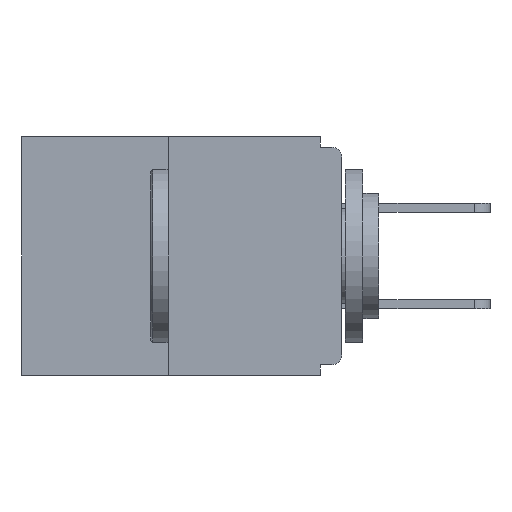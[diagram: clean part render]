
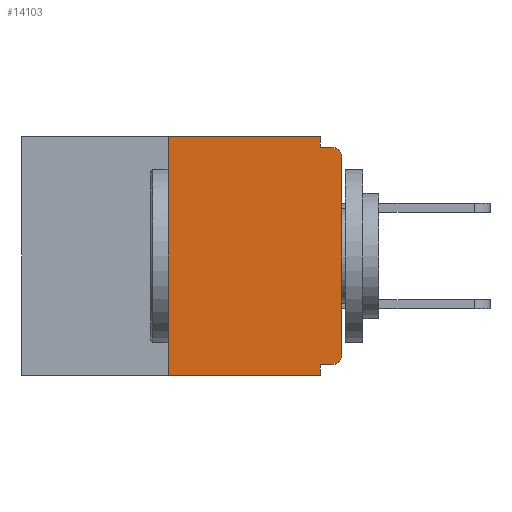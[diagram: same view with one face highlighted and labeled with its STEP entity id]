
A CAD part, left-side view. The second image highlights one B-rep face of the part: STEP entity #14103.
In plain terms, the highlighted planar face has unit normal (-1, 0, 0).
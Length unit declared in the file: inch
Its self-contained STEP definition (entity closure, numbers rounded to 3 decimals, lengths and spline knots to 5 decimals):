
#642 = CARTESIAN_POINT ( 'NONE',  ( 0., 0., 0. ) ) ;
#660 = CIRCLE ( 'NONE', #4347, 0.015 ) ;
#723 = VECTOR ( 'NONE', #12560, 39.37008 ) ;
#788 = EDGE_CURVE ( 'NONE', #7187, #11592, #7968, .T. ) ;
#806 = ORIENTED_EDGE ( 'NONE', *, *, #14814, .F. ) ;
#1246 = EDGE_CURVE ( 'NONE', #4702, #4030, #9407, .T. ) ;
#1365 = DIRECTION ( 'NONE',  ( 0., 0., -1. ) ) ;
#1454 = CARTESIAN_POINT ( 'NONE',  ( 0., 0.031, -0.328 ) ) ;
#1514 = DIRECTION ( 'NONE',  ( 0., 0., -1. ) ) ;
#1721 = VECTOR ( 'NONE', #4648, 39.37008 ) ;
#2261 = CARTESIAN_POINT ( 'NONE',  ( 0., 0.015, -0.03 ) ) ;
#2440 = VECTOR ( 'NONE', #11767, 39.37008 ) ;
#2476 = CARTESIAN_POINT ( 'NONE',  ( 0., 0.031, -0.343 ) ) ;
#2668 = DIRECTION ( 'NONE',  ( 0., 0., -1. ) ) ;
#3034 = LINE ( 'NONE', #5674, #2440 ) ;
#3120 = VECTOR ( 'NONE', #1514, 39.37008 ) ;
#3167 = ORIENTED_EDGE ( 'NONE', *, *, #3266, .T. ) ;
#3266 = EDGE_CURVE ( 'NONE', #11592, #13795, #10700, .T. ) ;
#3483 = DIRECTION ( 'NONE',  ( 0., 0., -1. ) ) ;
#3600 = ORIENTED_EDGE ( 'NONE', *, *, #12355, .F. ) ;
#3883 = DIRECTION ( 'NONE',  ( 0., -1., 0. ) ) ;
#4005 = VERTEX_POINT ( 'NONE', #1454 ) ;
#4030 = VERTEX_POINT ( 'NONE', #2476 ) ;
#4347 = AXIS2_PLACEMENT_3D ( 'NONE', #14617, #5137, #1365 ) ;
#4400 = LINE ( 'NONE', #5538, #4951 ) ;
#4648 = DIRECTION ( 'NONE',  ( 0., 1., 0. ) ) ;
#4702 = VERTEX_POINT ( 'NONE', #8155 ) ;
#4951 = VECTOR ( 'NONE', #5646, 39.37008 ) ;
#4954 = CARTESIAN_POINT ( 'NONE',  ( 0., 0.46, 0. ) ) ;
#5137 = DIRECTION ( 'NONE',  ( -1., 0., 0. ) ) ;
#5209 = EDGE_CURVE ( 'NONE', #8473, #13795, #3034, .T. ) ;
#5538 = CARTESIAN_POINT ( 'NONE',  ( 0., 0.25, 0. ) ) ;
#5549 = FACE_OUTER_BOUND ( 'NONE', #7481, .T. ) ;
#5646 = DIRECTION ( 'NONE',  ( 0., 0., 1. ) ) ;
#5674 = CARTESIAN_POINT ( 'NONE',  ( 0., 0., -0.015 ) ) ;
#5801 = VECTOR ( 'NONE', #3883, 39.37008 ) ;
#5940 = VERTEX_POINT ( 'NONE', #10066 ) ;
#6025 = AXIS2_PLACEMENT_3D ( 'NONE', #4954, #13485, #6295 ) ;
#6147 = CARTESIAN_POINT ( 'NONE',  ( 0., 0.031, 0. ) ) ;
#6292 = VECTOR ( 'NONE', #13688, 39.37008 ) ;
#6295 = DIRECTION ( 'NONE',  ( 0., 0., -1. ) ) ;
#6958 = EDGE_CURVE ( 'NONE', #7143, #7187, #660, .T. ) ;
#7143 = VERTEX_POINT ( 'NONE', #15646 ) ;
#7187 = VERTEX_POINT ( 'NONE', #8089 ) ;
#7480 = ORIENTED_EDGE ( 'NONE', *, *, #12812, .F. ) ;
#7481 = EDGE_LOOP ( 'NONE', ( #7480, #3600, #12255, #13884, #806, #10613, #14303, #3167, #12494, #14920 ) ) ;
#7607 = LINE ( 'NONE', #8601, #9303 ) ;
#7968 = LINE ( 'NONE', #642, #723 ) ;
#8089 = CARTESIAN_POINT ( 'NONE',  ( 0., 0., -0.313 ) ) ;
#8155 = CARTESIAN_POINT ( 'NONE',  ( 0., 0.25, -0.343 ) ) ;
#8163 = CARTESIAN_POINT ( 'NONE',  ( 0., 0., -0.328 ) ) ;
#8193 = LINE ( 'NONE', #8163, #1721 ) ;
#8228 = VERTEX_POINT ( 'NONE', #6147 ) ;
#8473 = VERTEX_POINT ( 'NONE', #10403 ) ;
#8601 = CARTESIAN_POINT ( 'NONE',  ( 0., 0.031, -0.343 ) ) ;
#8856 = CARTESIAN_POINT ( 'NONE',  ( 0., 0.031, 0. ) ) ;
#9303 = VECTOR ( 'NONE', #2668, 39.37008 ) ;
#9407 = LINE ( 'NONE', #11268, #5801 ) ;
#10066 = CARTESIAN_POINT ( 'NONE',  ( 0., 0.25, 0. ) ) ;
#10297 = AXIS2_PLACEMENT_3D ( 'NONE', #2261, #13179, #3483 ) ;
#10403 = CARTESIAN_POINT ( 'NONE',  ( 0., 0.031, -0.015 ) ) ;
#10613 = ORIENTED_EDGE ( 'NONE', *, *, #6958, .T. ) ;
#10700 = CIRCLE ( 'NONE', #10297, 0.015 ) ;
#11166 = EDGE_CURVE ( 'NONE', #8228, #8473, #12918, .T. ) ;
#11233 = LINE ( 'NONE', #12457, #6292 ) ;
#11268 = CARTESIAN_POINT ( 'NONE',  ( 0., 0.46, -0.343 ) ) ;
#11592 = VERTEX_POINT ( 'NONE', #14993 ) ;
#11767 = DIRECTION ( 'NONE',  ( 0., -1., 0. ) ) ;
#12114 = CARTESIAN_POINT ( 'NONE',  ( 0., 0.015, -0.015 ) ) ;
#12205 = PLANE ( 'NONE',  #6025 ) ;
#12255 = ORIENTED_EDGE ( 'NONE', *, *, #1246, .T. ) ;
#12355 = EDGE_CURVE ( 'NONE', #4702, #5940, #4400, .T. ) ;
#12457 = CARTESIAN_POINT ( 'NONE',  ( 0., 0.46, 0. ) ) ;
#12494 = ORIENTED_EDGE ( 'NONE', *, *, #5209, .F. ) ;
#12560 = DIRECTION ( 'NONE',  ( 0., 0., 1. ) ) ;
#12812 = EDGE_CURVE ( 'NONE', #5940, #8228, #11233, .T. ) ;
#12918 = LINE ( 'NONE', #8856, #3120 ) ;
#13179 = DIRECTION ( 'NONE',  ( -1., 0., 0. ) ) ;
#13283 = EDGE_CURVE ( 'NONE', #4005, #4030, #7607, .T. ) ;
#13485 = DIRECTION ( 'NONE',  ( 1., 0., 0. ) ) ;
#13688 = DIRECTION ( 'NONE',  ( 0., -1., 0. ) ) ;
#13795 = VERTEX_POINT ( 'NONE', #12114 ) ;
#13884 = ORIENTED_EDGE ( 'NONE', *, *, #13283, .F. ) ;
#14103 = ADVANCED_FACE ( 'NONE', ( #5549 ), #12205, .F. ) ;
#14303 = ORIENTED_EDGE ( 'NONE', *, *, #788, .T. ) ;
#14617 = CARTESIAN_POINT ( 'NONE',  ( 0., 0.015, -0.313 ) ) ;
#14814 = EDGE_CURVE ( 'NONE', #7143, #4005, #8193, .T. ) ;
#14920 = ORIENTED_EDGE ( 'NONE', *, *, #11166, .F. ) ;
#14993 = CARTESIAN_POINT ( 'NONE',  ( 0., 0., -0.03 ) ) ;
#15646 = CARTESIAN_POINT ( 'NONE',  ( 0., 0.015, -0.328 ) ) ;
